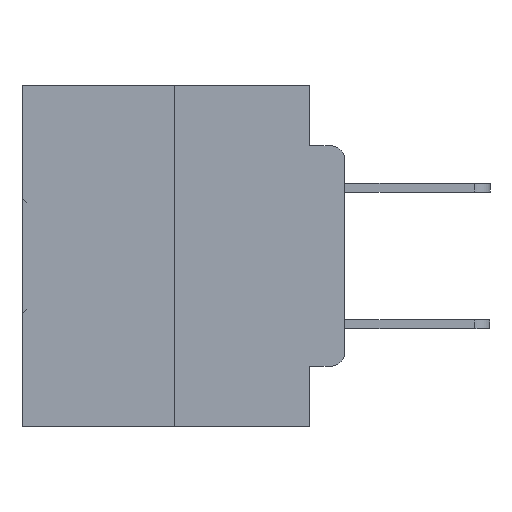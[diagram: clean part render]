
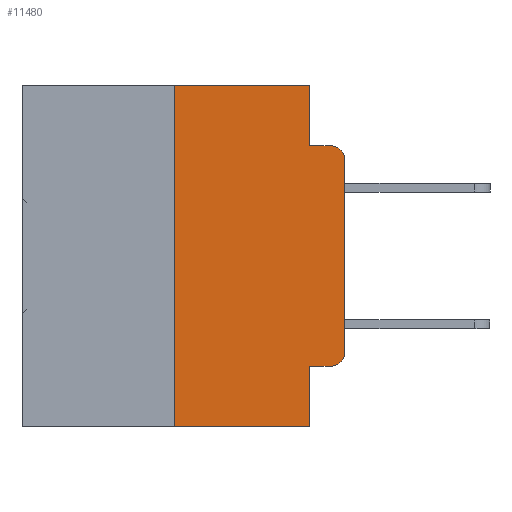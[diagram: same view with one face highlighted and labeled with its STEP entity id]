
A CAD part, left-side view. The second image highlights one B-rep face of the part: STEP entity #11480.
In plain terms, the highlighted planar face has unit normal (-1, 0, 0).
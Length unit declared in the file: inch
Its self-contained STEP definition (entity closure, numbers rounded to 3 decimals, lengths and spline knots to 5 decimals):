
#123 = CARTESIAN_POINT ( 'NONE',  ( 0., 0.051, -0.5 ) ) ;
#215 = CARTESIAN_POINT ( 'NONE',  ( 0., 0., -0.3915 ) ) ;
#447 = CARTESIAN_POINT ( 'NONE',  ( 0., 0.25, -0.5 ) ) ;
#754 = LINE ( 'NONE', #19179, #14436 ) ;
#1645 = LINE ( 'NONE', #21850, #21280 ) ;
#2730 = VECTOR ( 'NONE', #15727, 39.37008 ) ;
#2892 = EDGE_CURVE ( 'NONE', #22716, #12116, #16004, .T. ) ;
#3022 = FACE_OUTER_BOUND ( 'NONE', #32449, .T. ) ;
#3102 = EDGE_CURVE ( 'NONE', #7425, #27057, #16384, .T. ) ;
#3252 = CARTESIAN_POINT ( 'NONE',  ( 0., 0.473, 0. ) ) ;
#3287 = DIRECTION ( 'NONE',  ( 0., -1., 0. ) ) ;
#3477 = CARTESIAN_POINT ( 'NONE',  ( 0., 0.02, -0.3915 ) ) ;
#3647 = ORIENTED_EDGE ( 'NONE', *, *, #15692, .F. ) ;
#3972 = DIRECTION ( 'NONE',  ( 0., 0., 1. ) ) ;
#4035 = ORIENTED_EDGE ( 'NONE', *, *, #13341, .T. ) ;
#4063 = ORIENTED_EDGE ( 'NONE', *, *, #7154, .F. ) ;
#4275 = VERTEX_POINT ( 'NONE', #19369 ) ;
#4472 = ORIENTED_EDGE ( 'NONE', *, *, #14064, .T. ) ;
#4743 = EDGE_CURVE ( 'NONE', #32478, #9653, #20245, .T. ) ;
#5294 = CIRCLE ( 'NONE', #11572, 0.02 ) ;
#5699 = AXIS2_PLACEMENT_3D ( 'NONE', #28471, #13255, #31048 ) ;
#6096 = DIRECTION ( 'NONE',  ( 0., 0., -1. ) ) ;
#7154 = EDGE_CURVE ( 'NONE', #30498, #22716, #1645, .T. ) ;
#7425 = VERTEX_POINT ( 'NONE', #17719 ) ;
#7577 = CARTESIAN_POINT ( 'NONE',  ( 0., 0.02, -0.0885 ) ) ;
#8853 = EDGE_CURVE ( 'NONE', #11101, #23881, #26743, .T. ) ;
#8935 = CARTESIAN_POINT ( 'NONE',  ( 0., 0.051, -0.0885 ) ) ;
#9592 = DIRECTION ( 'NONE',  ( 1., 0., 0. ) ) ;
#9653 = VERTEX_POINT ( 'NONE', #7577 ) ;
#9770 = LINE ( 'NONE', #31902, #15734 ) ;
#10988 = LINE ( 'NONE', #12570, #16991 ) ;
#11020 = CIRCLE ( 'NONE', #5699, 0.02 ) ;
#11101 = VERTEX_POINT ( 'NONE', #215 ) ;
#11480 = ADVANCED_FACE ( 'NONE', ( #3022 ), #19732, .F. ) ;
#11572 = AXIS2_PLACEMENT_3D ( 'NONE', #3477, #21373, #6096 ) ;
#12102 = ORIENTED_EDGE ( 'NONE', *, *, #2892, .F. ) ;
#12116 = VERTEX_POINT ( 'NONE', #32535 ) ;
#12476 = ORIENTED_EDGE ( 'NONE', *, *, #4743, .F. ) ;
#12570 = CARTESIAN_POINT ( 'NONE',  ( 0., 0.473, -0.5 ) ) ;
#13255 = DIRECTION ( 'NONE',  ( -1., 0., 0. ) ) ;
#13341 = EDGE_CURVE ( 'NONE', #23881, #9653, #11020, .T. ) ;
#13808 = EDGE_CURVE ( 'NONE', #30498, #27057, #10988, .T. ) ;
#13875 = CARTESIAN_POINT ( 'NONE',  ( 0., 0.051, -0.0885 ) ) ;
#14064 = EDGE_CURVE ( 'NONE', #7425, #4275, #9770, .T. ) ;
#14221 = DIRECTION ( 'NONE',  ( 0., -1., 0. ) ) ;
#14436 = VECTOR ( 'NONE', #21716, 39.37008 ) ;
#15692 = EDGE_CURVE ( 'NONE', #12116, #32478, #754, .T. ) ;
#15727 = DIRECTION ( 'NONE',  ( 0., 0., -1. ) ) ;
#15734 = VECTOR ( 'NONE', #21809, 39.37008 ) ;
#16004 = LINE ( 'NONE', #3252, #21970 ) ;
#16084 = DIRECTION ( 'NONE',  ( 0., 0., 1. ) ) ;
#16384 = LINE ( 'NONE', #20750, #2730 ) ;
#16582 = AXIS2_PLACEMENT_3D ( 'NONE', #17176, #9592, #27380 ) ;
#16991 = VECTOR ( 'NONE', #30369, 39.37008 ) ;
#17176 = CARTESIAN_POINT ( 'NONE',  ( 0., 0.473, 0. ) ) ;
#17258 = ORIENTED_EDGE ( 'NONE', *, *, #8853, .T. ) ;
#17719 = CARTESIAN_POINT ( 'NONE',  ( 0., 0.051, -0.4115 ) ) ;
#18909 = ORIENTED_EDGE ( 'NONE', *, *, #22159, .T. ) ;
#19030 = CARTESIAN_POINT ( 'NONE',  ( 0., 0.25, 0. ) ) ;
#19179 = CARTESIAN_POINT ( 'NONE',  ( 0., 0.051, 0. ) ) ;
#19369 = CARTESIAN_POINT ( 'NONE',  ( 0., 0.02, -0.4115 ) ) ;
#19732 = PLANE ( 'NONE',  #16582 ) ;
#20245 = LINE ( 'NONE', #13875, #32912 ) ;
#20750 = CARTESIAN_POINT ( 'NONE',  ( 0., 0.051, 0. ) ) ;
#21280 = VECTOR ( 'NONE', #3972, 39.37008 ) ;
#21373 = DIRECTION ( 'NONE',  ( -1., 0., 0. ) ) ;
#21716 = DIRECTION ( 'NONE',  ( 0., 0., -1. ) ) ;
#21809 = DIRECTION ( 'NONE',  ( 0., -1., 0. ) ) ;
#21850 = CARTESIAN_POINT ( 'NONE',  ( 0., 0.25, 0. ) ) ;
#21970 = VECTOR ( 'NONE', #3287, 39.37008 ) ;
#22159 = EDGE_CURVE ( 'NONE', #4275, #11101, #5294, .T. ) ;
#22716 = VERTEX_POINT ( 'NONE', #19030 ) ;
#23481 = CARTESIAN_POINT ( 'NONE',  ( 0., 0., -0.1085 ) ) ;
#23881 = VERTEX_POINT ( 'NONE', #23481 ) ;
#26743 = LINE ( 'NONE', #28719, #32657 ) ;
#26855 = ORIENTED_EDGE ( 'NONE', *, *, #3102, .F. ) ;
#27057 = VERTEX_POINT ( 'NONE', #123 ) ;
#27380 = DIRECTION ( 'NONE',  ( 0., 0., -1. ) ) ;
#28471 = CARTESIAN_POINT ( 'NONE',  ( 0., 0.02, -0.1085 ) ) ;
#28719 = CARTESIAN_POINT ( 'NONE',  ( 0., 0., 0. ) ) ;
#30369 = DIRECTION ( 'NONE',  ( 0., -1., 0. ) ) ;
#30498 = VERTEX_POINT ( 'NONE', #447 ) ;
#31048 = DIRECTION ( 'NONE',  ( 0., 0., -1. ) ) ;
#31902 = CARTESIAN_POINT ( 'NONE',  ( 0., 0.051, -0.4115 ) ) ;
#31990 = ORIENTED_EDGE ( 'NONE', *, *, #13808, .T. ) ;
#32449 = EDGE_LOOP ( 'NONE', ( #17258, #4035, #12476, #3647, #12102, #4063, #31990, #26855, #4472, #18909 ) ) ;
#32478 = VERTEX_POINT ( 'NONE', #8935 ) ;
#32535 = CARTESIAN_POINT ( 'NONE',  ( 0., 0.051, 0. ) ) ;
#32657 = VECTOR ( 'NONE', #16084, 39.37008 ) ;
#32912 = VECTOR ( 'NONE', #14221, 39.37008 ) ;
